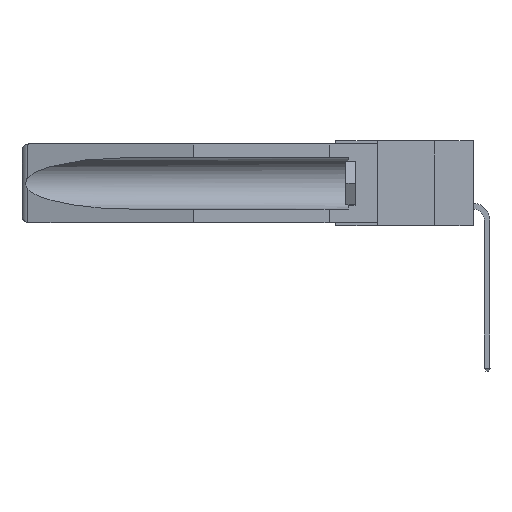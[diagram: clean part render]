
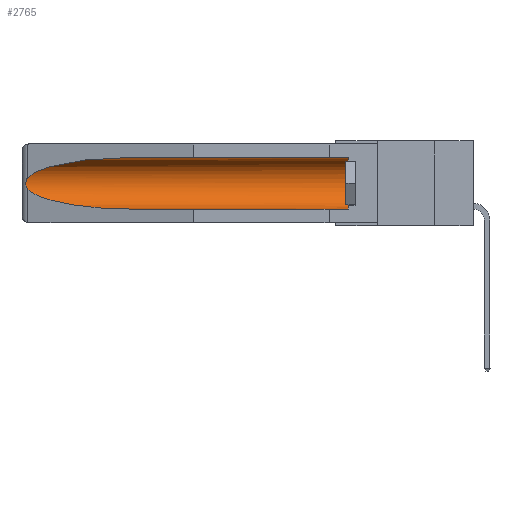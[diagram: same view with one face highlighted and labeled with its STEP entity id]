
A CAD part, left-side view. The second image highlights one B-rep face of the part: STEP entity #2765.
In plain terms, the highlighted cylindrical face has radius 2.857 mm (diameter 5.715 mm), a partial arc.
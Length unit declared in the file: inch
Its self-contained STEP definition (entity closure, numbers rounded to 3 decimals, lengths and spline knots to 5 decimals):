
#773 = ORIENTED_EDGE ( 'NONE', *, *, #7630, .F. ) ;
#855 = CARTESIAN_POINT ( 'NONE',  ( 0.155, 1.07973, -0.284 ) ) ;
#1186 = CARTESIAN_POINT ( 'NONE',  ( 0.26597, 1.5296, -0.19026 ) ) ;
#1328 = VERTEX_POINT ( 'NONE', #10772 ) ;
#1788 = CARTESIAN_POINT ( 'NONE',  ( 0.25451, 1.48313, -0.09465 ) ) ;
#2093 = CARTESIAN_POINT ( 'NONE',  ( 0.26654, 1.53092, -0.15636 ) ) ;
#2120 = CIRCLE ( 'NONE', #11669, 0.1125 ) ;
#2327 = ORIENTED_EDGE ( 'NONE', *, *, #12622, .T. ) ;
#2622 = DIRECTION ( 'NONE',  ( 0., 0., 1. ) ) ;
#2765 = ADVANCED_FACE ( 'NONE', ( #3776 ), #3560, .F. ) ;
#3126 = VERTEX_POINT ( 'NONE', #15618 ) ;
#3416 = CARTESIAN_POINT ( 'NONE',  ( 0.155, -0.30754, -0.284 ) ) ;
#3560 = CYLINDRICAL_SURFACE ( 'NONE', #10885, 0.1125 ) ;
#3576 = VECTOR ( 'NONE', #8191, 39.37008 ) ;
#3610 = CARTESIAN_POINT ( 'NONE',  ( 0.26537, 1.52718, -0.14972 ) ) ;
#3776 = FACE_OUTER_BOUND ( 'NONE', #13044, .T. ) ;
#3880 = VECTOR ( 'NONE', #8334, 39.37008 ) ;
#4500 =( BOUNDED_CURVE ( )  B_SPLINE_CURVE ( 3, ( #13886, #6557, #6749, #855 ),
 .UNSPECIFIED., .F., .F. ) 
 B_SPLINE_CURVE_WITH_KNOTS ( ( 4, 4 ),
 ( 0.1948, 1.5708 ),
 .UNSPECIFIED. ) 
 CURVE ( )  GEOMETRIC_REPRESENTATION_ITEM ( )  RATIONAL_B_SPLINE_CURVE ( ( 1., 0.848, 0.848, 1. ) ) 
 REPRESENTATION_ITEM ( '' )  );
#4985 = CARTESIAN_POINT ( 'NONE',  ( 0.155, 0.126, -0.284 ) ) ;
#5096 = CARTESIAN_POINT ( 'NONE',  ( 0.155, -0.30754, -0.059 ) ) ;
#5307 = VERTEX_POINT ( 'NONE', #11152 ) ;
#5378 = ORIENTED_EDGE ( 'NONE', *, *, #5882, .T. ) ;
#5503 = CARTESIAN_POINT ( 'NONE',  ( 0.155, 0.126, -0.1715 ) ) ;
#5882 = EDGE_CURVE ( 'NONE', #6047, #5307, #14501, .T. ) ;
#6047 = VERTEX_POINT ( 'NONE', #14072 ) ;
#6557 = CARTESIAN_POINT ( 'NONE',  ( 0.25451, 1.48313, -0.24835 ) ) ;
#6642 = CARTESIAN_POINT ( 'NONE',  ( 0.2673, 1.53269, -0.17917 ) ) ;
#6749 = CARTESIAN_POINT ( 'NONE',  ( 0.21114, 1.30732, -0.284 ) ) ;
#7400 = LINE ( 'NONE', #3416, #3576 ) ;
#7630 = EDGE_CURVE ( 'NONE', #10227, #1328, #7400, .T. ) ;
#8191 = DIRECTION ( 'NONE',  ( 0., 1., 0. ) ) ;
#8334 = DIRECTION ( 'NONE',  ( 0., 1., 0. ) ) ;
#9922 = DIRECTION ( 'NONE',  ( 0., -1., 0. ) ) ;
#10091 = DIRECTION ( 'NONE',  ( 0., 0., 1. ) ) ;
#10227 = VERTEX_POINT ( 'NONE', #4985 ) ;
#10335 = EDGE_CURVE ( 'NONE', #10227, #13093, #2120, .T. ) ;
#10506 = ORIENTED_EDGE ( 'NONE', *, *, #10335, .T. ) ;
#10772 = CARTESIAN_POINT ( 'NONE',  ( 0.155, 1.07973, -0.284 ) ) ;
#10885 = AXIS2_PLACEMENT_3D ( 'NONE', #14308, #13074, #10091 ) ;
#11067 = ORIENTED_EDGE ( 'NONE', *, *, #17836, .T. ) ;
#11152 = CARTESIAN_POINT ( 'NONE',  ( 0.26537, 1.52718, -0.14972 ) ) ;
#11591 = CARTESIAN_POINT ( 'NONE',  ( 0.26537, 1.52718, -0.19328 ) ) ;
#11669 = AXIS2_PLACEMENT_3D ( 'NONE', #5503, #9922, #2622 ) ;
#12622 = EDGE_CURVE ( 'NONE', #13093, #6047, #14882, .T. ) ;
#12924 = EDGE_CURVE ( 'NONE', #5307, #3126, #17579, .T. ) ;
#13044 = EDGE_LOOP ( 'NONE', ( #5378, #13197, #11067, #773, #10506, #2327 ) ) ;
#13074 = DIRECTION ( 'NONE',  ( 0., 1., 0. ) ) ;
#13093 = VERTEX_POINT ( 'NONE', #18146 ) ;
#13197 = ORIENTED_EDGE ( 'NONE', *, *, #12924, .T. ) ;
#13886 = CARTESIAN_POINT ( 'NONE',  ( 0.26537, 1.52718, -0.19328 ) ) ;
#14046 = CARTESIAN_POINT ( 'NONE',  ( 0.2675, 1.53308, -0.16763 ) ) ;
#14072 = CARTESIAN_POINT ( 'NONE',  ( 0.155, 1.07973, -0.059 ) ) ;
#14308 = CARTESIAN_POINT ( 'NONE',  ( 0.155, -0.30754, -0.1715 ) ) ;
#14501 =( BOUNDED_CURVE ( )  B_SPLINE_CURVE ( 3, ( #14539, #14604, #1788, #17359 ),
 .UNSPECIFIED., .F., .F. ) 
 B_SPLINE_CURVE_WITH_KNOTS ( ( 4, 4 ),
 ( 4.71239, 6.08839 ),
 .UNSPECIFIED. ) 
 CURVE ( )  GEOMETRIC_REPRESENTATION_ITEM ( )  RATIONAL_B_SPLINE_CURVE ( ( 1., 0.848, 0.848, 1. ) ) 
 REPRESENTATION_ITEM ( '' )  );
#14539 = CARTESIAN_POINT ( 'NONE',  ( 0.155, 1.07973, -0.059 ) ) ;
#14599 = CARTESIAN_POINT ( 'NONE',  ( 0.26655, 1.53094, -0.18657 ) ) ;
#14604 = CARTESIAN_POINT ( 'NONE',  ( 0.21114, 1.30732, -0.059 ) ) ;
#14882 = LINE ( 'NONE', #5096, #3880 ) ;
#15206 = CARTESIAN_POINT ( 'NONE',  ( 0.2675, 1.53308, -0.17534 ) ) ;
#15618 = CARTESIAN_POINT ( 'NONE',  ( 0.26537, 1.52718, -0.19328 ) ) ;
#16406 = CARTESIAN_POINT ( 'NONE',  ( 0.26597, 1.52961, -0.15275 ) ) ;
#16717 = CARTESIAN_POINT ( 'NONE',  ( 0.2673, 1.5327, -0.16383 ) ) ;
#17359 = CARTESIAN_POINT ( 'NONE',  ( 0.26537, 1.52718, -0.14972 ) ) ;
#17579 = B_SPLINE_CURVE_WITH_KNOTS ( 'NONE', 3,
 ( #3610, #16406, #2093, #16717, #14046, #15206, #6642, #14599, #1186, #11591 ),
 .UNSPECIFIED., .F., .F.,
 ( 4, 2, 2, 2, 4 ),
 ( 0., 0.00029, 0.00058, 0.00087, 0.00117 ),
 .UNSPECIFIED. ) ;
#17836 = EDGE_CURVE ( 'NONE', #3126, #1328, #4500, .T. ) ;
#18146 = CARTESIAN_POINT ( 'NONE',  ( 0.155, 0.126, -0.059 ) ) ;
